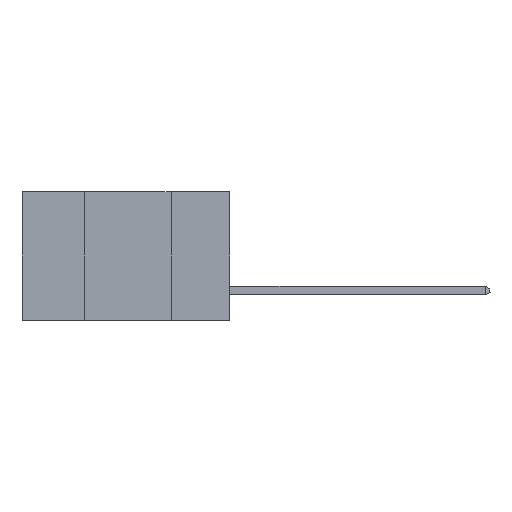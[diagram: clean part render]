
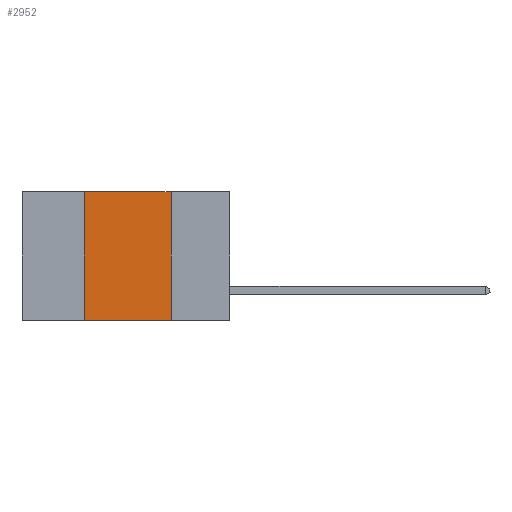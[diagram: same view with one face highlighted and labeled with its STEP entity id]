
A CAD part, left-side view. The second image highlights one B-rep face of the part: STEP entity #2952.
In plain terms, the highlighted planar face has unit normal (-1, 0, 0).
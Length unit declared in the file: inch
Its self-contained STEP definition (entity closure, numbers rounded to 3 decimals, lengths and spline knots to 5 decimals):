
#734 = DIRECTION ( 'NONE',  ( 0., -1., 0. ) ) ;
#912 = CARTESIAN_POINT ( 'NONE',  ( 0., 0.42, 0. ) ) ;
#951 = LINE ( 'NONE', #4760, #14871 ) ;
#1010 = VECTOR ( 'NONE', #6827, 39.37008 ) ;
#1143 = EDGE_CURVE ( 'NONE', #5588, #14904, #8962, .T. ) ;
#1620 = ORIENTED_EDGE ( 'NONE', *, *, #14498, .F. ) ;
#1655 = VERTEX_POINT ( 'NONE', #912 ) ;
#1747 = LINE ( 'NONE', #13807, #1010 ) ;
#2343 = DIRECTION ( 'NONE',  ( 0., 0., -1. ) ) ;
#2952 = ADVANCED_FACE ( 'NONE', ( #13598 ), #6041, .F. ) ;
#3288 = AXIS2_PLACEMENT_3D ( 'NONE', #14206, #14319, #11934 ) ;
#4275 = ORIENTED_EDGE ( 'NONE', *, *, #1143, .T. ) ;
#4760 = CARTESIAN_POINT ( 'NONE',  ( 0., 0.17, 0. ) ) ;
#5349 = ORIENTED_EDGE ( 'NONE', *, *, #11077, .F. ) ;
#5588 = VERTEX_POINT ( 'NONE', #9447 ) ;
#6041 = PLANE ( 'NONE',  #3288 ) ;
#6827 = DIRECTION ( 'NONE',  ( 0., 0., 1. ) ) ;
#8602 = VECTOR ( 'NONE', #13594, 39.37008 ) ;
#8645 = EDGE_CURVE ( 'NONE', #1655, #13889, #9684, .T. ) ;
#8962 = LINE ( 'NONE', #13802, #8602 ) ;
#9447 = CARTESIAN_POINT ( 'NONE',  ( 0., 0.42, -0.37 ) ) ;
#9604 = ORIENTED_EDGE ( 'NONE', *, *, #8645, .F. ) ;
#9684 = LINE ( 'NONE', #12372, #11163 ) ;
#9895 = CARTESIAN_POINT ( 'NONE',  ( 0., 0.17, -0.37 ) ) ;
#10597 = CARTESIAN_POINT ( 'NONE',  ( 0., 0.17, 0. ) ) ;
#11077 = EDGE_CURVE ( 'NONE', #5588, #1655, #1747, .T. ) ;
#11163 = VECTOR ( 'NONE', #734, 39.37008 ) ;
#11934 = DIRECTION ( 'NONE',  ( 0., 0., -1. ) ) ;
#12372 = CARTESIAN_POINT ( 'NONE',  ( 0., 0.6, 0. ) ) ;
#13143 = EDGE_LOOP ( 'NONE', ( #1620, #9604, #5349, #4275 ) ) ;
#13594 = DIRECTION ( 'NONE',  ( 0., -1., 0. ) ) ;
#13598 = FACE_OUTER_BOUND ( 'NONE', #13143, .T. ) ;
#13802 = CARTESIAN_POINT ( 'NONE',  ( 0., 0.6, -0.37 ) ) ;
#13807 = CARTESIAN_POINT ( 'NONE',  ( 0., 0.42, 0. ) ) ;
#13889 = VERTEX_POINT ( 'NONE', #10597 ) ;
#14206 = CARTESIAN_POINT ( 'NONE',  ( 0., 0.6, 0. ) ) ;
#14319 = DIRECTION ( 'NONE',  ( 1., 0., 0. ) ) ;
#14498 = EDGE_CURVE ( 'NONE', #13889, #14904, #951, .T. ) ;
#14871 = VECTOR ( 'NONE', #2343, 39.37008 ) ;
#14904 = VERTEX_POINT ( 'NONE', #9895 ) ;
